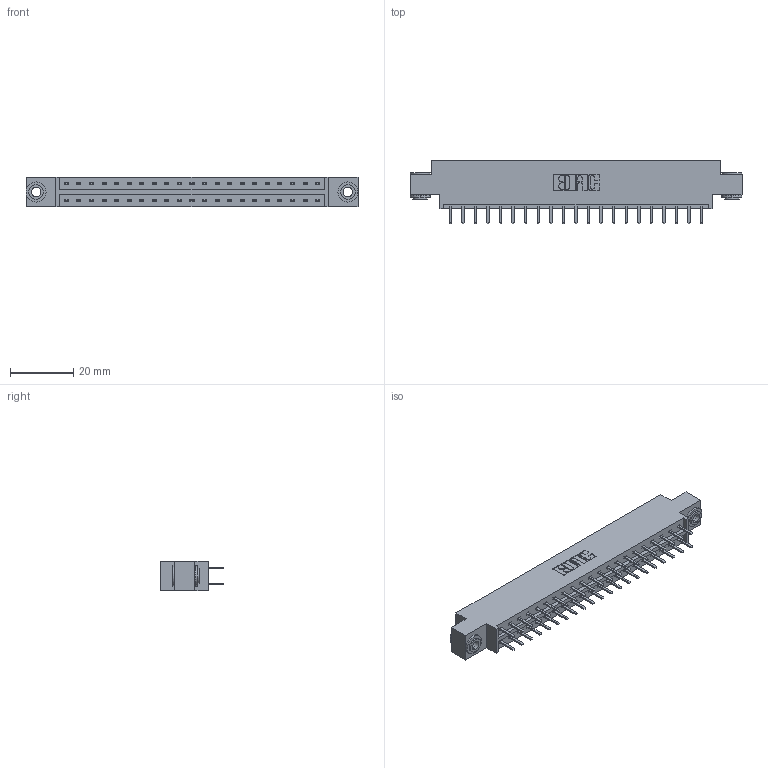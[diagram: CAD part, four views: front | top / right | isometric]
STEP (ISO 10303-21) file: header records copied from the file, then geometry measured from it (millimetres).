
FILE_DESCRIPTION (( 'STEP AP203' ), '1' );
FILE_NAME ('833-042-520-803.STEP', '2020-06-03T20:19:30', ( '' ), ( '' ), 'SwSTEP 2.0', 'SolidWorks 2020', '' );
FILE_SCHEMA (( 'CONFIG_CONTROL_DESIGN' ));
Length unit declared in the file: inch
Products named in the file (4): 833-042-520-803; 345-250-002_345-250-002-102; 345-292-001_345-293-120; 833 Part_Offset - .156 Dia - TH
Assembly tree (45 placements, depth 2):
  833-042-520-803
    833 Part_Offset - .156 Dia - TH
    345-292-001_345-293-120  x42
    345-250-002_345-250-002-102  x2
Bounding box: 104.75 x 20.02 x 9.4 mm (x, y, z)
Volume: 10271.1 mm3; surface area: 12310.1 mm2
Topology: 45 solids, 45 shells, 2508 faces, 7245 edges, 4714 vertices
Faces by surface type: plane 1680, cylinder 820, cone 8
Entity records: 17122 total; most frequent: CARTESIAN_POINT 2853, ORIENTED_EDGE 2770, DIRECTION 2495, EDGE_CURVE 1385, LINE 1229, VECTOR 1229, VERTEX_POINT 918, AXIS2_PLACEMENT_3D 633
